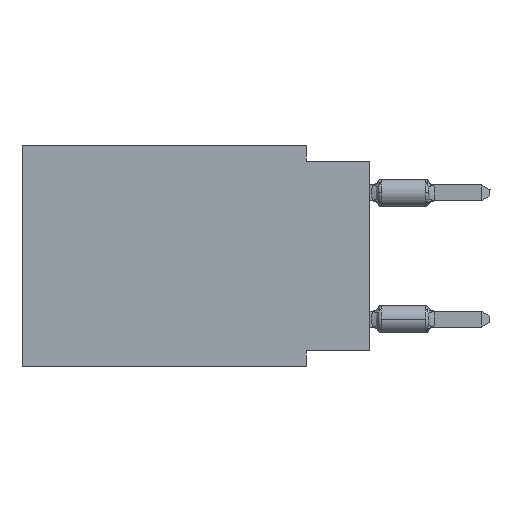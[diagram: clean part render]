
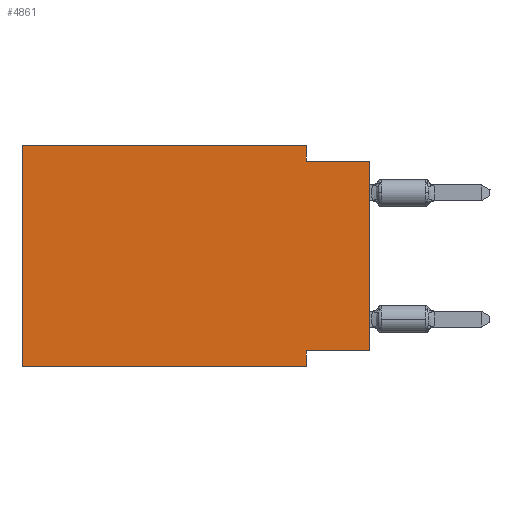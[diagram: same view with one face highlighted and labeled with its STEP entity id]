
A CAD part, left-side view. The second image highlights one B-rep face of the part: STEP entity #4861.
In plain terms, the highlighted planar face has unit normal (-1, 0, 0).
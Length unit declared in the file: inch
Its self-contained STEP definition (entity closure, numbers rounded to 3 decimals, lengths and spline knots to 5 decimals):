
#57 = DIRECTION ( 'NONE',  ( 0., 0., -1. ) ) ;
#75 = EDGE_CURVE ( 'NONE', #26498, #1994, #12143, .T. ) ;
#832 = CARTESIAN_POINT ( 'NONE',  ( 0., 0., 0. ) ) ;
#1076 = VERTEX_POINT ( 'NONE', #9078 ) ;
#1124 = DIRECTION ( 'NONE',  ( 0., 0., 1. ) ) ;
#1266 = EDGE_CURVE ( 'NONE', #1076, #26498, #9809, .T. ) ;
#1404 = LINE ( 'NONE', #832, #4483 ) ;
#1864 = VERTEX_POINT ( 'NONE', #9293 ) ;
#1994 = VERTEX_POINT ( 'NONE', #6794 ) ;
#2364 = CARTESIAN_POINT ( 'NONE',  ( 0., 0., -0.025 ) ) ;
#2534 = DIRECTION ( 'NONE',  ( 1., 0., 0. ) ) ;
#2934 = VERTEX_POINT ( 'NONE', #27623 ) ;
#2953 = ORIENTED_EDGE ( 'NONE', *, *, #28750, .T. ) ;
#3092 = ORIENTED_EDGE ( 'NONE', *, *, #75, .F. ) ;
#3184 = CARTESIAN_POINT ( 'NONE',  ( 0., 0.1, -0.35 ) ) ;
#3456 = DIRECTION ( 'NONE',  ( 0., 0., 1. ) ) ;
#3741 = VECTOR ( 'NONE', #4609, 39.37008 ) ;
#4141 = CARTESIAN_POINT ( 'NONE',  ( 0., 0.55, 0. ) ) ;
#4483 = VECTOR ( 'NONE', #1124, 39.37008 ) ;
#4609 = DIRECTION ( 'NONE',  ( 0., 0., -1. ) ) ;
#4771 = EDGE_LOOP ( 'NONE', ( #2953, #15049, #9049, #12076, #13874, #28790, #3092, #6576 ) ) ;
#4861 = ADVANCED_FACE ( 'NONE', ( #11200 ), #20133, .F. ) ;
#4895 = EDGE_CURVE ( 'NONE', #11958, #1994, #18808, .T. ) ;
#4901 = CARTESIAN_POINT ( 'NONE',  ( 0., 0.1, 0. ) ) ;
#5814 = DIRECTION ( 'NONE',  ( 0., 1., 0. ) ) ;
#6576 = ORIENTED_EDGE ( 'NONE', *, *, #1266, .F. ) ;
#6794 = CARTESIAN_POINT ( 'NONE',  ( 0., 0.1, -0.35 ) ) ;
#7364 = CARTESIAN_POINT ( 'NONE',  ( 0., 0.55, -0.35 ) ) ;
#8153 = LINE ( 'NONE', #28185, #21901 ) ;
#9049 = ORIENTED_EDGE ( 'NONE', *, *, #13531, .F. ) ;
#9078 = CARTESIAN_POINT ( 'NONE',  ( 0., 0., -0.325 ) ) ;
#9191 = CARTESIAN_POINT ( 'NONE',  ( 0., 0.55, -0.35 ) ) ;
#9293 = CARTESIAN_POINT ( 'NONE',  ( 0., 0.1, -0.025 ) ) ;
#9607 = VECTOR ( 'NONE', #5814, 39.37008 ) ;
#9809 = LINE ( 'NONE', #12427, #9607 ) ;
#9839 = VECTOR ( 'NONE', #25591, 39.37008 ) ;
#11135 = CARTESIAN_POINT ( 'NONE',  ( 0., 0., -0.025 ) ) ;
#11200 = FACE_OUTER_BOUND ( 'NONE', #4771, .T. ) ;
#11667 = LINE ( 'NONE', #4901, #3741 ) ;
#11958 = VERTEX_POINT ( 'NONE', #9191 ) ;
#12076 = ORIENTED_EDGE ( 'NONE', *, *, #16184, .F. ) ;
#12143 = LINE ( 'NONE', #3184, #9839 ) ;
#12297 = VECTOR ( 'NONE', #16749, 39.37008 ) ;
#12316 = VECTOR ( 'NONE', #15980, 39.37008 ) ;
#12427 = CARTESIAN_POINT ( 'NONE',  ( 0., 0., -0.325 ) ) ;
#13531 = EDGE_CURVE ( 'NONE', #28212, #1864, #11667, .T. ) ;
#13874 = ORIENTED_EDGE ( 'NONE', *, *, #17987, .F. ) ;
#14423 = AXIS2_PLACEMENT_3D ( 'NONE', #4141, #2534, #57 ) ;
#14696 = LINE ( 'NONE', #23654, #12297 ) ;
#15049 = ORIENTED_EDGE ( 'NONE', *, *, #24874, .F. ) ;
#15980 = DIRECTION ( 'NONE',  ( 0., -1., 0. ) ) ;
#16184 = EDGE_CURVE ( 'NONE', #2934, #28212, #14696, .T. ) ;
#16446 = DIRECTION ( 'NONE',  ( 0., -1., 0. ) ) ;
#16749 = DIRECTION ( 'NONE',  ( 0., -1., 0. ) ) ;
#17987 = EDGE_CURVE ( 'NONE', #11958, #2934, #8153, .T. ) ;
#18175 = VECTOR ( 'NONE', #16446, 39.37008 ) ;
#18808 = LINE ( 'NONE', #7364, #18175 ) ;
#20133 = PLANE ( 'NONE',  #14423 ) ;
#21901 = VECTOR ( 'NONE', #3456, 39.37008 ) ;
#23641 = CARTESIAN_POINT ( 'NONE',  ( 0., 0.1, 0. ) ) ;
#23654 = CARTESIAN_POINT ( 'NONE',  ( 0., 0.55, 0. ) ) ;
#23967 = CARTESIAN_POINT ( 'NONE',  ( 0., 0.1, -0.325 ) ) ;
#24874 = EDGE_CURVE ( 'NONE', #1864, #25452, #28449, .T. ) ;
#25452 = VERTEX_POINT ( 'NONE', #11135 ) ;
#25591 = DIRECTION ( 'NONE',  ( 0., 0., -1. ) ) ;
#26498 = VERTEX_POINT ( 'NONE', #23967 ) ;
#27623 = CARTESIAN_POINT ( 'NONE',  ( 0., 0.55, 0. ) ) ;
#28185 = CARTESIAN_POINT ( 'NONE',  ( 0., 0.55, 0. ) ) ;
#28212 = VERTEX_POINT ( 'NONE', #23641 ) ;
#28449 = LINE ( 'NONE', #2364, #12316 ) ;
#28750 = EDGE_CURVE ( 'NONE', #1076, #25452, #1404, .T. ) ;
#28790 = ORIENTED_EDGE ( 'NONE', *, *, #4895, .T. ) ;
